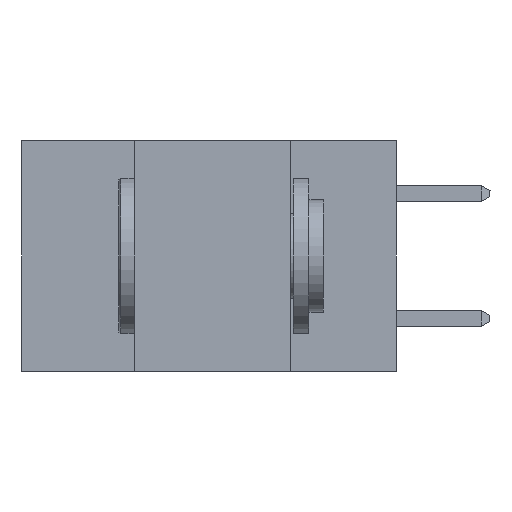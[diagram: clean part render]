
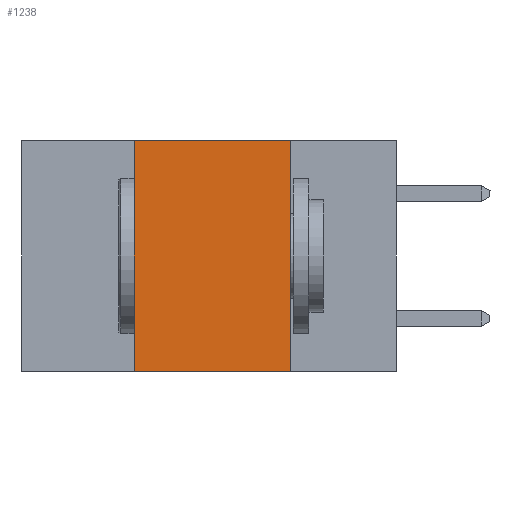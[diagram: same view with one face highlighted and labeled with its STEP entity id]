
A CAD part, left-side view. The second image highlights one B-rep face of the part: STEP entity #1238.
In plain terms, the highlighted planar face has unit normal (-1, 0, 0).
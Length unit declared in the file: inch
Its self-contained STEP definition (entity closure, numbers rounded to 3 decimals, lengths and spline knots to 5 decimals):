
#292 = ORIENTED_EDGE ( 'NONE', *, *, #5926, .T. ) ;
#1238 = ADVANCED_FACE ( 'NONE', ( #11993 ), #26007, .F. ) ;
#1408 = VERTEX_POINT ( 'NONE', #9316 ) ;
#2640 = LINE ( 'NONE', #12873, #19359 ) ;
#3579 = LINE ( 'NONE', #12450, #25799 ) ;
#4486 = CARTESIAN_POINT ( 'NONE',  ( 0., 0.17, -0.37 ) ) ;
#5926 = EDGE_CURVE ( 'NONE', #9087, #8344, #3579, .T. ) ;
#6082 = VECTOR ( 'NONE', #6618, 39.37008 ) ;
#6618 = DIRECTION ( 'NONE',  ( 0., 0., -1. ) ) ;
#7353 = EDGE_CURVE ( 'NONE', #9087, #9360, #2640, .T. ) ;
#8344 = VERTEX_POINT ( 'NONE', #24413 ) ;
#8470 = DIRECTION ( 'NONE',  ( 0., -1., 0. ) ) ;
#9087 = VERTEX_POINT ( 'NONE', #19040 ) ;
#9316 = CARTESIAN_POINT ( 'NONE',  ( 0., 0.17, 0. ) ) ;
#9360 = VERTEX_POINT ( 'NONE', #15673 ) ;
#10428 = ORIENTED_EDGE ( 'NONE', *, *, #13297, .F. ) ;
#11797 = EDGE_CURVE ( 'NONE', #9360, #1408, #14411, .T. ) ;
#11993 = FACE_OUTER_BOUND ( 'NONE', #16116, .T. ) ;
#12450 = CARTESIAN_POINT ( 'NONE',  ( 0., 0.6, -0.37 ) ) ;
#12873 = CARTESIAN_POINT ( 'NONE',  ( 0., 0.42, -0.37 ) ) ;
#13297 = EDGE_CURVE ( 'NONE', #1408, #8344, #23364, .T. ) ;
#14411 = LINE ( 'NONE', #14884, #25021 ) ;
#14884 = CARTESIAN_POINT ( 'NONE',  ( 0., 0.6, 0. ) ) ;
#15673 = CARTESIAN_POINT ( 'NONE',  ( 0., 0.42, 0. ) ) ;
#16116 = EDGE_LOOP ( 'NONE', ( #10428, #20975, #24109, #292 ) ) ;
#18675 = AXIS2_PLACEMENT_3D ( 'NONE', #27308, #25771, #25735 ) ;
#19040 = CARTESIAN_POINT ( 'NONE',  ( 0., 0.42, -0.37 ) ) ;
#19208 = DIRECTION ( 'NONE',  ( 0., -1., 0. ) ) ;
#19359 = VECTOR ( 'NONE', #19407, 39.37008 ) ;
#19407 = DIRECTION ( 'NONE',  ( 0., 0., 1. ) ) ;
#20975 = ORIENTED_EDGE ( 'NONE', *, *, #11797, .F. ) ;
#23364 = LINE ( 'NONE', #4486, #6082 ) ;
#24109 = ORIENTED_EDGE ( 'NONE', *, *, #7353, .F. ) ;
#24413 = CARTESIAN_POINT ( 'NONE',  ( 0., 0.17, -0.37 ) ) ;
#25021 = VECTOR ( 'NONE', #19208, 39.37008 ) ;
#25735 = DIRECTION ( 'NONE',  ( 0., 0., -1. ) ) ;
#25771 = DIRECTION ( 'NONE',  ( 1., 0., 0. ) ) ;
#25799 = VECTOR ( 'NONE', #8470, 39.37008 ) ;
#26007 = PLANE ( 'NONE',  #18675 ) ;
#27308 = CARTESIAN_POINT ( 'NONE',  ( 0., 0.6, 0. ) ) ;
